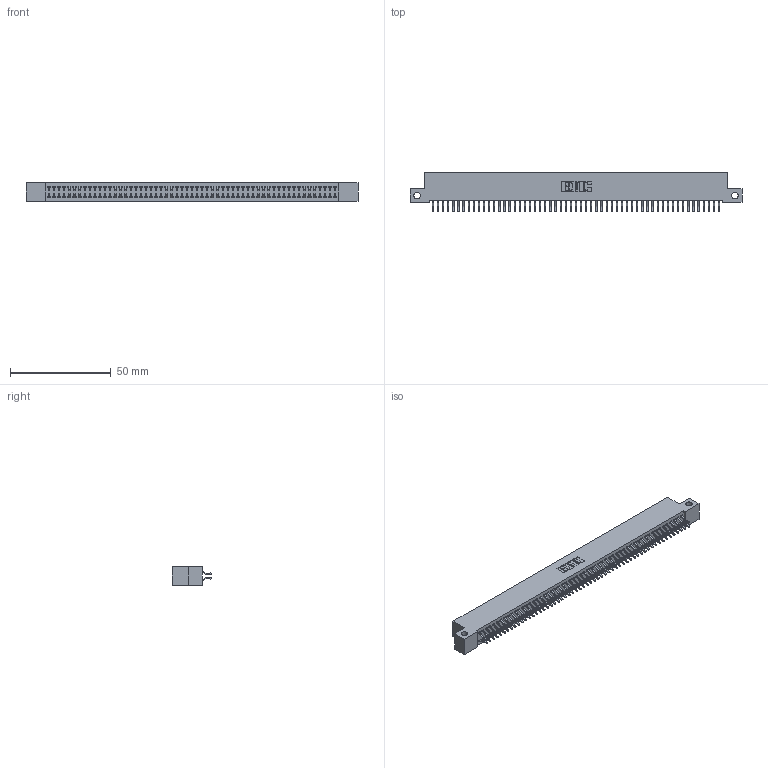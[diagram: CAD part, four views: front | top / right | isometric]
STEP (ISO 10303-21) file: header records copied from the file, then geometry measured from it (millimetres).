
FILE_DESCRIPTION (( 'STEP AP203' ), '1' );
FILE_NAME ('342-114-556-212.STEP', '2018-08-14T13:10:11', ( '' ), ( '' ), 'SwSTEP 2.0', 'SolidWorks 2016', '' );
FILE_SCHEMA (( 'CONFIG_CONTROL_DESIGN' ));
Length unit declared in the file: inch
Products named in the file (3): 342 Part_Side Mount; 345-292-001_556 Tail; 342-114-556-212
Assembly tree (115 placements, depth 2):
  342-114-556-212
    342 Part_Side Mount
    345-292-001_556 Tail  x114
Bounding box: 165.1 x 19.58 x 9.4 mm (x, y, z)
Volume: 14828.4 mm3; surface area: 24236.2 mm2
Topology: 115 solids, 115 shells, 6722 faces, 20021 edges, 13194 vertices
Faces by surface type: plane 4626, cylinder 2096
Entity records: 34821 total; most frequent: CARTESIAN_POINT 5766, ORIENTED_EDGE 5690, DIRECTION 4889, EDGE_CURVE 2845, LINE 2709, VECTOR 2709, VERTEX_POINT 1894, AXIS2_PLACEMENT_3D 1090
